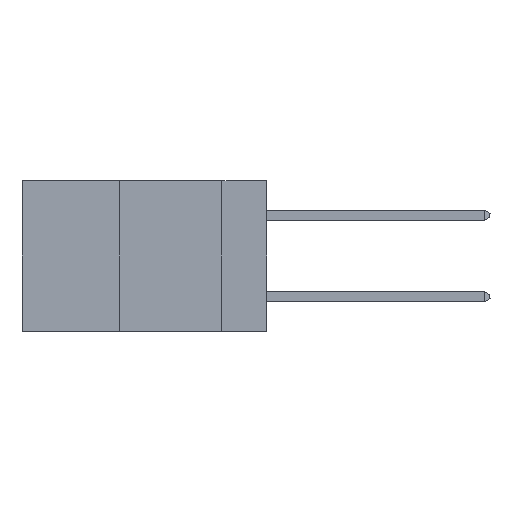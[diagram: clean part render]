
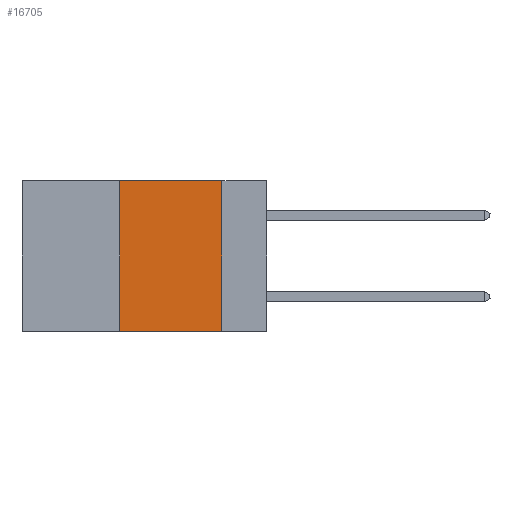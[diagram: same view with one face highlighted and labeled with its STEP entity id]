
A CAD part, left-side view. The second image highlights one B-rep face of the part: STEP entity #16705.
In plain terms, the highlighted planar face has unit normal (-1, 0, 0).
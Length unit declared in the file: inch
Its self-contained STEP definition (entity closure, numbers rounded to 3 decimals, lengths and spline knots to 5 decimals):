
#4578 = ORIENTED_EDGE ( 'NONE', *, *, #28945, .T. ) ;
#5684 = LINE ( 'NONE', #19134, #36741 ) ;
#6367 = ORIENTED_EDGE ( 'NONE', *, *, #32712, .F. ) ;
#6937 = CARTESIAN_POINT ( 'NONE',  ( 0., 0.11, 0. ) ) ;
#7217 = LINE ( 'NONE', #12088, #9087 ) ;
#7591 = VERTEX_POINT ( 'NONE', #6937 ) ;
#9087 = VECTOR ( 'NONE', #34003, 39.37008 ) ;
#9159 = DIRECTION ( 'NONE',  ( 1., 0., 0. ) ) ;
#10088 = VECTOR ( 'NONE', #22085, 39.37008 ) ;
#11171 = CARTESIAN_POINT ( 'NONE',  ( 0., 0.36, 0. ) ) ;
#12088 = CARTESIAN_POINT ( 'NONE',  ( 0., 0.11, 0. ) ) ;
#13450 = CARTESIAN_POINT ( 'NONE',  ( 0., 0.11, -0.37 ) ) ;
#13952 = VERTEX_POINT ( 'NONE', #11171 ) ;
#16180 = CARTESIAN_POINT ( 'NONE',  ( 0., 0.6, -0.37 ) ) ;
#16705 = ADVANCED_FACE ( 'NONE', ( #21573 ), #18561, .F. ) ;
#18427 = DIRECTION ( 'NONE',  ( 0., 0., -1. ) ) ;
#18561 = PLANE ( 'NONE',  #34550 ) ;
#19134 = CARTESIAN_POINT ( 'NONE',  ( 0., 0.6, 0. ) ) ;
#21312 = VERTEX_POINT ( 'NONE', #38177 ) ;
#21573 = FACE_OUTER_BOUND ( 'NONE', #30500, .T. ) ;
#22085 = DIRECTION ( 'NONE',  ( 0., -1., 0. ) ) ;
#23664 = ORIENTED_EDGE ( 'NONE', *, *, #35639, .F. ) ;
#25167 = CARTESIAN_POINT ( 'NONE',  ( 0., 0.36, 0. ) ) ;
#26353 = ORIENTED_EDGE ( 'NONE', *, *, #26813, .F. ) ;
#26813 = EDGE_CURVE ( 'NONE', #7591, #33822, #7217, .T. ) ;
#27209 = CARTESIAN_POINT ( 'NONE',  ( 0., 0.6, 0. ) ) ;
#27272 = LINE ( 'NONE', #25167, #32845 ) ;
#28945 = EDGE_CURVE ( 'NONE', #21312, #33822, #35506, .T. ) ;
#30500 = EDGE_LOOP ( 'NONE', ( #26353, #23664, #6367, #4578 ) ) ;
#32712 = EDGE_CURVE ( 'NONE', #21312, #13952, #27272, .T. ) ;
#32845 = VECTOR ( 'NONE', #34181, 39.37008 ) ;
#33822 = VERTEX_POINT ( 'NONE', #13450 ) ;
#34003 = DIRECTION ( 'NONE',  ( 0., 0., -1. ) ) ;
#34181 = DIRECTION ( 'NONE',  ( 0., 0., 1. ) ) ;
#34550 = AXIS2_PLACEMENT_3D ( 'NONE', #27209, #9159, #18427 ) ;
#35506 = LINE ( 'NONE', #16180, #10088 ) ;
#35639 = EDGE_CURVE ( 'NONE', #13952, #7591, #5684, .T. ) ;
#36704 = DIRECTION ( 'NONE',  ( 0., -1., 0. ) ) ;
#36741 = VECTOR ( 'NONE', #36704, 39.37008 ) ;
#38177 = CARTESIAN_POINT ( 'NONE',  ( 0., 0.36, -0.37 ) ) ;
